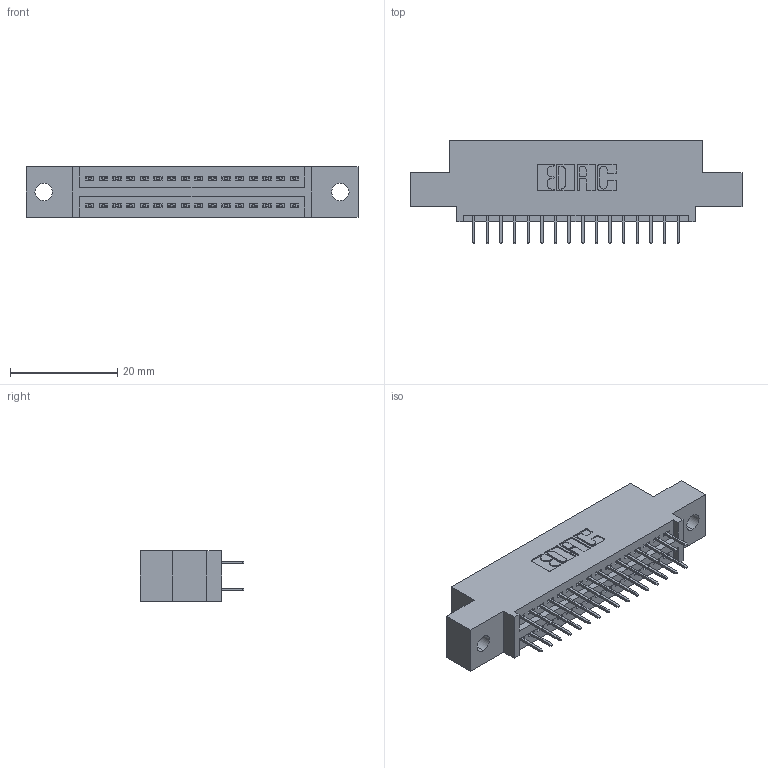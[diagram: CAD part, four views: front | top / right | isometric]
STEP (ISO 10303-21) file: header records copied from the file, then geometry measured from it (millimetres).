
FILE_DESCRIPTION (( 'STEP AP203' ), '1' );
FILE_NAME ('345-032-524-502.STEP', '2019-10-28T03:54:03', ( '' ), ( '' ), 'SwSTEP 2.0', 'SolidWorks 2016', '' );
FILE_SCHEMA (( 'CONFIG_CONTROL_DESIGN' ));
Length unit declared in the file: inch
Products named in the file (3): 345 Part_0.110 Offset - 0.128 Dia; 345-032-524-502; 345-292-001_345-293-124
Assembly tree (33 placements, depth 2):
  345-032-524-502
    345 Part_0.110 Offset - 0.128 Dia
    345-292-001_345-293-124  x32
Bounding box: 61.85 x 19.35 x 9.4 mm (x, y, z)
Volume: 5608.3 mm3; surface area: 7478.7 mm2
Topology: 33 solids, 33 shells, 1858 faces, 5249 edges, 3370 vertices
Faces by surface type: plane 1332, cylinder 526
Entity records: 16263 total; most frequent: CARTESIAN_POINT 2752, ORIENTED_EDGE 2686, DIRECTION 2459, EDGE_CURVE 1343, LINE 1151, VECTOR 1151, VERTEX_POINT 890, AXIS2_PLACEMENT_3D 654
